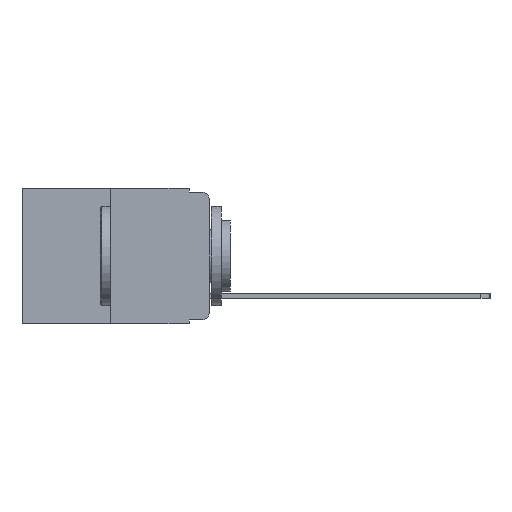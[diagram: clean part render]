
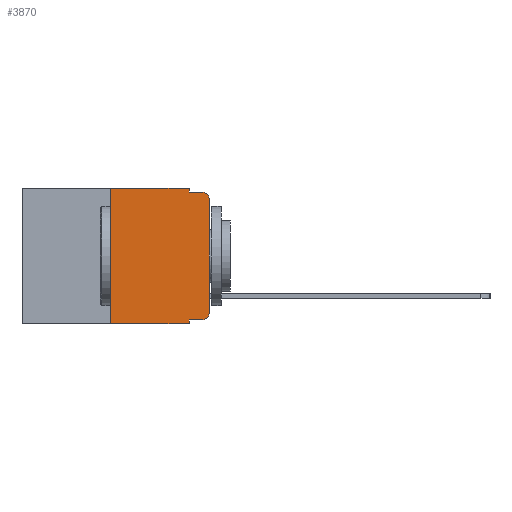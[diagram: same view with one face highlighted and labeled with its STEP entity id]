
A CAD part, left-side view. The second image highlights one B-rep face of the part: STEP entity #3870.
In plain terms, the highlighted planar face has unit normal (-1, 0, 0).
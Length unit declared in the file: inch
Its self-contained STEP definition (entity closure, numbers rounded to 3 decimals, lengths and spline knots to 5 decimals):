
#8 = VECTOR ( 'NONE', #4091, 39.37008 ) ;
#104 = CARTESIAN_POINT ( 'NONE',  ( 0., 0.473, 0. ) ) ;
#145 = DIRECTION ( 'NONE',  ( 1., 0., 0. ) ) ;
#701 = LINE ( 'NONE', #4247, #8332 ) ;
#811 = VECTOR ( 'NONE', #3212, 39.37008 ) ;
#984 = CIRCLE ( 'NONE', #10611, 0.02 ) ;
#1317 = CARTESIAN_POINT ( 'NONE',  ( 0., 0., -0.313 ) ) ;
#1507 = VECTOR ( 'NONE', #5295, 39.37008 ) ;
#1807 = LINE ( 'NONE', #9913, #11666 ) ;
#2132 = DIRECTION ( 'NONE',  ( 0., -1., 0. ) ) ;
#2457 = LINE ( 'NONE', #11346, #4890 ) ;
#2564 = CARTESIAN_POINT ( 'NONE',  ( 0., 0.051, -0.01 ) ) ;
#3010 = CARTESIAN_POINT ( 'NONE',  ( 0., 0.25, -0.343 ) ) ;
#3033 = CARTESIAN_POINT ( 'NONE',  ( 0., 0.051, -0.333 ) ) ;
#3173 = DIRECTION ( 'NONE',  ( -1., 0., 0. ) ) ;
#3212 = DIRECTION ( 'NONE',  ( 0., -1., 0. ) ) ;
#3216 = DIRECTION ( 'NONE',  ( 0., 0., 1. ) ) ;
#3273 = AXIS2_PLACEMENT_3D ( 'NONE', #104, #145, #7228 ) ;
#3768 = CARTESIAN_POINT ( 'NONE',  ( 0., 0.051, 0. ) ) ;
#3870 = ADVANCED_FACE ( 'NONE', ( #4952 ), #4324, .F. ) ;
#3949 = LINE ( 'NONE', #11733, #11079 ) ;
#3976 = CARTESIAN_POINT ( 'NONE',  ( 0., 0.02, -0.01 ) ) ;
#4027 = CARTESIAN_POINT ( 'NONE',  ( 0., 0., -0.03 ) ) ;
#4043 = CARTESIAN_POINT ( 'NONE',  ( 0., 0.051, -0.01 ) ) ;
#4091 = DIRECTION ( 'NONE',  ( 0., -1., 0. ) ) ;
#4247 = CARTESIAN_POINT ( 'NONE',  ( 0., 0.473, 0. ) ) ;
#4324 = PLANE ( 'NONE',  #3273 ) ;
#4365 = DIRECTION ( 'NONE',  ( 0., 0., -1. ) ) ;
#4439 = VECTOR ( 'NONE', #11108, 39.37008 ) ;
#4676 = VERTEX_POINT ( 'NONE', #3010 ) ;
#4791 = DIRECTION ( 'NONE',  ( -1., 0., 0. ) ) ;
#4890 = VECTOR ( 'NONE', #4920, 39.37008 ) ;
#4904 = CIRCLE ( 'NONE', #5924, 0.02 ) ;
#4920 = DIRECTION ( 'NONE',  ( 0., 0., 1. ) ) ;
#4952 = FACE_OUTER_BOUND ( 'NONE', #9956, .T. ) ;
#4988 = VERTEX_POINT ( 'NONE', #11743 ) ;
#5295 = DIRECTION ( 'NONE',  ( 0., 0., -1. ) ) ;
#5437 = EDGE_CURVE ( 'NONE', #4988, #10660, #10414, .T. ) ;
#5488 = EDGE_CURVE ( 'NONE', #10660, #8403, #4904, .T. ) ;
#5518 = EDGE_CURVE ( 'NONE', #4676, #9399, #1807, .T. ) ;
#5543 = EDGE_CURVE ( 'NONE', #4988, #12432, #6845, .T. ) ;
#5575 = EDGE_CURVE ( 'NONE', #6639, #11037, #3949, .T. ) ;
#5589 = ORIENTED_EDGE ( 'NONE', *, *, #5969, .T. ) ;
#5764 = EDGE_CURVE ( 'NONE', #11037, #12190, #6691, .T. ) ;
#5862 = EDGE_CURVE ( 'NONE', #9730, #12190, #984, .T. ) ;
#5924 = AXIS2_PLACEMENT_3D ( 'NONE', #8970, #3173, #9876 ) ;
#5926 = ORIENTED_EDGE ( 'NONE', *, *, #5862, .T. ) ;
#5969 = EDGE_CURVE ( 'NONE', #8403, #9730, #2457, .T. ) ;
#6118 = ORIENTED_EDGE ( 'NONE', *, *, #5764, .F. ) ;
#6190 = ORIENTED_EDGE ( 'NONE', *, *, #5575, .F. ) ;
#6639 = VERTEX_POINT ( 'NONE', #3768 ) ;
#6667 = ORIENTED_EDGE ( 'NONE', *, *, #8216, .F. ) ;
#6691 = LINE ( 'NONE', #2564, #4439 ) ;
#6759 = ORIENTED_EDGE ( 'NONE', *, *, #5518, .F. ) ;
#6785 = ORIENTED_EDGE ( 'NONE', *, *, #6962, .T. ) ;
#6845 = LINE ( 'NONE', #8117, #1507 ) ;
#6962 = EDGE_CURVE ( 'NONE', #4676, #12432, #10810, .T. ) ;
#7141 = CARTESIAN_POINT ( 'NONE',  ( 0., 0.473, -0.343 ) ) ;
#7192 = ORIENTED_EDGE ( 'NONE', *, *, #5543, .F. ) ;
#7202 = ORIENTED_EDGE ( 'NONE', *, *, #5437, .T. ) ;
#7228 = DIRECTION ( 'NONE',  ( 0., 0., -1. ) ) ;
#7367 = ORIENTED_EDGE ( 'NONE', *, *, #5488, .T. ) ;
#8117 = CARTESIAN_POINT ( 'NONE',  ( 0., 0.051, 0. ) ) ;
#8128 = CARTESIAN_POINT ( 'NONE',  ( 0., 0.051, -0.343 ) ) ;
#8216 = EDGE_CURVE ( 'NONE', #9399, #6639, #701, .T. ) ;
#8332 = VECTOR ( 'NONE', #2132, 39.37008 ) ;
#8403 = VERTEX_POINT ( 'NONE', #1317 ) ;
#8970 = CARTESIAN_POINT ( 'NONE',  ( 0., 0.02, -0.313 ) ) ;
#9399 = VERTEX_POINT ( 'NONE', #12025 ) ;
#9730 = VERTEX_POINT ( 'NONE', #4027 ) ;
#9876 = DIRECTION ( 'NONE',  ( 0., 0., -1. ) ) ;
#9913 = CARTESIAN_POINT ( 'NONE',  ( 0., 0.25, 0. ) ) ;
#9956 = EDGE_LOOP ( 'NONE', ( #5589, #5926, #6118, #6190, #6667, #6759, #6785, #7192, #7202, #7367 ) ) ;
#10326 = CARTESIAN_POINT ( 'NONE',  ( 0., 0.02, -0.333 ) ) ;
#10355 = CARTESIAN_POINT ( 'NONE',  ( 0., 0.02, -0.03 ) ) ;
#10414 = LINE ( 'NONE', #3033, #8 ) ;
#10611 = AXIS2_PLACEMENT_3D ( 'NONE', #10355, #4791, #11235 ) ;
#10660 = VERTEX_POINT ( 'NONE', #10326 ) ;
#10810 = LINE ( 'NONE', #7141, #811 ) ;
#11037 = VERTEX_POINT ( 'NONE', #4043 ) ;
#11079 = VECTOR ( 'NONE', #4365, 39.37008 ) ;
#11108 = DIRECTION ( 'NONE',  ( 0., -1., 0. ) ) ;
#11235 = DIRECTION ( 'NONE',  ( 0., 0., -1. ) ) ;
#11346 = CARTESIAN_POINT ( 'NONE',  ( 0., 0., 0. ) ) ;
#11666 = VECTOR ( 'NONE', #3216, 39.37008 ) ;
#11733 = CARTESIAN_POINT ( 'NONE',  ( 0., 0.051, 0. ) ) ;
#11743 = CARTESIAN_POINT ( 'NONE',  ( 0., 0.051, -0.333 ) ) ;
#12025 = CARTESIAN_POINT ( 'NONE',  ( 0., 0.25, 0. ) ) ;
#12190 = VERTEX_POINT ( 'NONE', #3976 ) ;
#12432 = VERTEX_POINT ( 'NONE', #8128 ) ;
